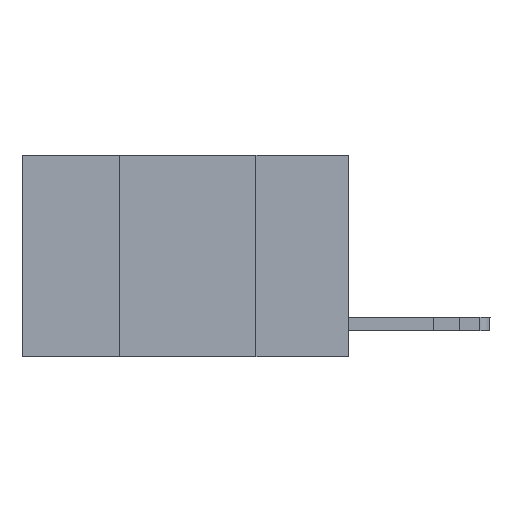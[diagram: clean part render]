
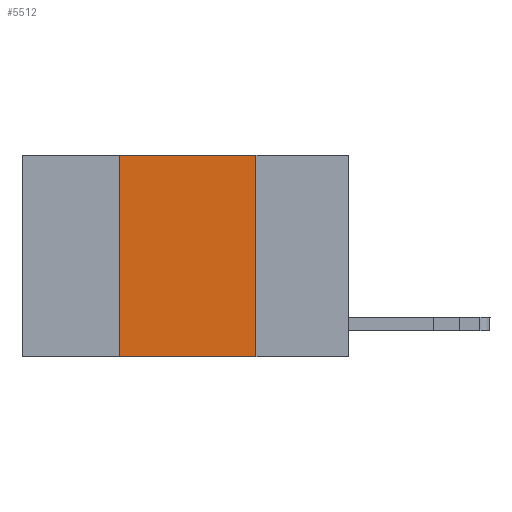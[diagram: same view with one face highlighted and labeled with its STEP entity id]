
A CAD part, left-side view. The second image highlights one B-rep face of the part: STEP entity #5512.
In plain terms, the highlighted planar face has unit normal (-1, 0, 0).
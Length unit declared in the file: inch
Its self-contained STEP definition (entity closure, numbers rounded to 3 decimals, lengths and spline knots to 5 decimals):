
#270 = VERTEX_POINT ( 'NONE', #7155 ) ;
#1114 = CARTESIAN_POINT ( 'NONE',  ( 0., 0.42, 0. ) ) ;
#1694 = LINE ( 'NONE', #8825, #11167 ) ;
#1969 = LINE ( 'NONE', #6344, #8132 ) ;
#2384 = DIRECTION ( 'NONE',  ( 0., 0., 1. ) ) ;
#4100 = VERTEX_POINT ( 'NONE', #15359 ) ;
#4543 = LINE ( 'NONE', #8472, #7789 ) ;
#4574 = LINE ( 'NONE', #8144, #7438 ) ;
#4943 = ORIENTED_EDGE ( 'NONE', *, *, #15441, .F. ) ;
#5107 = CARTESIAN_POINT ( 'NONE',  ( 0., 0.17, -0.37 ) ) ;
#5512 = ADVANCED_FACE ( 'NONE', ( #8548 ), #14672, .F. ) ;
#6292 = EDGE_CURVE ( 'NONE', #270, #13492, #4574, .T. ) ;
#6344 = CARTESIAN_POINT ( 'NONE',  ( 0., 0.17, 0. ) ) ;
#7080 = EDGE_CURVE ( 'NONE', #270, #8351, #4543, .T. ) ;
#7155 = CARTESIAN_POINT ( 'NONE',  ( 0., 0.42, -0.37 ) ) ;
#7386 = CARTESIAN_POINT ( 'NONE',  ( 0., 0.6, 0. ) ) ;
#7438 = VECTOR ( 'NONE', #9355, 39.37008 ) ;
#7532 = DIRECTION ( 'NONE',  ( 0., 0., -1. ) ) ;
#7789 = VECTOR ( 'NONE', #2384, 39.37008 ) ;
#7879 = EDGE_CURVE ( 'NONE', #4100, #13492, #1969, .T. ) ;
#8132 = VECTOR ( 'NONE', #7532, 39.37008 ) ;
#8144 = CARTESIAN_POINT ( 'NONE',  ( 0., 0.6, -0.37 ) ) ;
#8351 = VERTEX_POINT ( 'NONE', #1114 ) ;
#8472 = CARTESIAN_POINT ( 'NONE',  ( 0., 0.42, 0. ) ) ;
#8548 = FACE_OUTER_BOUND ( 'NONE', #9050, .T. ) ;
#8581 = DIRECTION ( 'NONE',  ( 0., 0., -1. ) ) ;
#8825 = CARTESIAN_POINT ( 'NONE',  ( 0., 0.6, 0. ) ) ;
#9050 = EDGE_LOOP ( 'NONE', ( #9190, #4943, #9378, #9410 ) ) ;
#9190 = ORIENTED_EDGE ( 'NONE', *, *, #7879, .F. ) ;
#9355 = DIRECTION ( 'NONE',  ( 0., -1., 0. ) ) ;
#9378 = ORIENTED_EDGE ( 'NONE', *, *, #7080, .F. ) ;
#9410 = ORIENTED_EDGE ( 'NONE', *, *, #6292, .T. ) ;
#10092 = DIRECTION ( 'NONE',  ( 0., -1., 0. ) ) ;
#11167 = VECTOR ( 'NONE', #10092, 39.37008 ) ;
#11178 = AXIS2_PLACEMENT_3D ( 'NONE', #7386, #15891, #8581 ) ;
#13492 = VERTEX_POINT ( 'NONE', #5107 ) ;
#14672 = PLANE ( 'NONE',  #11178 ) ;
#15359 = CARTESIAN_POINT ( 'NONE',  ( 0., 0.17, 0. ) ) ;
#15441 = EDGE_CURVE ( 'NONE', #8351, #4100, #1694, .T. ) ;
#15891 = DIRECTION ( 'NONE',  ( 1., 0., 0. ) ) ;
